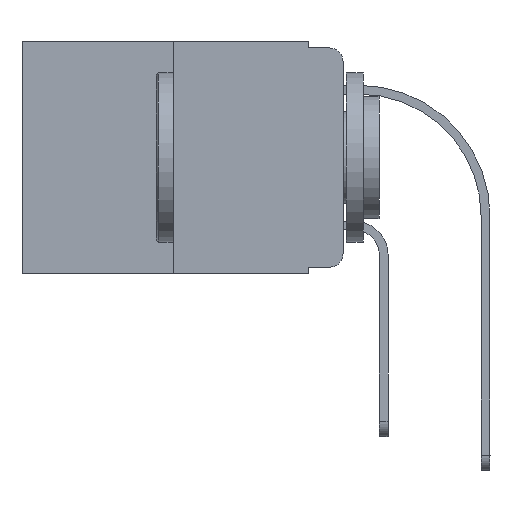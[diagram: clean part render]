
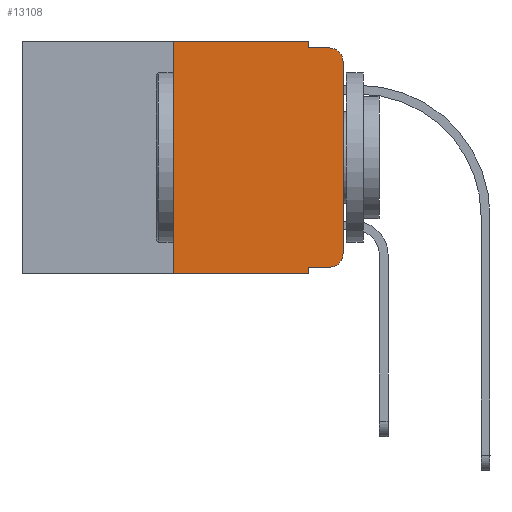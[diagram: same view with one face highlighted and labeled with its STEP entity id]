
A CAD part, left-side view. The second image highlights one B-rep face of the part: STEP entity #13108.
In plain terms, the highlighted planar face has unit normal (-1, 0, 0).
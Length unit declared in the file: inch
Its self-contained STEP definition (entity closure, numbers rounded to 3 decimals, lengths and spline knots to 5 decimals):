
#134 = DIRECTION ( 'NONE',  ( -1., 0., 0. ) ) ;
#656 = CARTESIAN_POINT ( 'NONE',  ( 0., 0., 0. ) ) ;
#934 = LINE ( 'NONE', #22986, #14768 ) ;
#983 = DIRECTION ( 'NONE',  ( 0., 0., -1. ) ) ;
#1268 = CARTESIAN_POINT ( 'NONE',  ( 0., 0.02, -0.01 ) ) ;
#1483 = VERTEX_POINT ( 'NONE', #3713 ) ;
#1506 = ORIENTED_EDGE ( 'NONE', *, *, #1952, .F. ) ;
#1589 = EDGE_CURVE ( 'NONE', #25586, #20872, #22453, .T. ) ;
#1952 = EDGE_CURVE ( 'NONE', #13489, #4452, #24661, .T. ) ;
#2121 = ORIENTED_EDGE ( 'NONE', *, *, #23318, .T. ) ;
#2332 = VERTEX_POINT ( 'NONE', #23731 ) ;
#2620 = DIRECTION ( 'NONE',  ( 0., -1., 0. ) ) ;
#2727 = DIRECTION ( 'NONE',  ( 0., -1., 0. ) ) ;
#2766 = CARTESIAN_POINT ( 'NONE',  ( 0., 0.051, -0.343 ) ) ;
#2879 = EDGE_CURVE ( 'NONE', #1483, #2332, #934, .T. ) ;
#3306 = ORIENTED_EDGE ( 'NONE', *, *, #19057, .F. ) ;
#3397 = VERTEX_POINT ( 'NONE', #7104 ) ;
#3544 = LINE ( 'NONE', #13345, #23094 ) ;
#3713 = CARTESIAN_POINT ( 'NONE',  ( 0., 0.051, -0.333 ) ) ;
#3762 = LINE ( 'NONE', #15770, #24955 ) ;
#3876 = FACE_OUTER_BOUND ( 'NONE', #21257, .T. ) ;
#3999 = CARTESIAN_POINT ( 'NONE',  ( 0., 0., -0.313 ) ) ;
#4319 = LINE ( 'NONE', #12385, #13441 ) ;
#4452 = VERTEX_POINT ( 'NONE', #1268 ) ;
#4532 = EDGE_CURVE ( 'NONE', #3397, #25586, #3762, .T. ) ;
#4614 = CARTESIAN_POINT ( 'NONE',  ( 0., 0.473, 0. ) ) ;
#6674 = CARTESIAN_POINT ( 'NONE',  ( 0., 0.25, 0. ) ) ;
#7056 = EDGE_CURVE ( 'NONE', #10008, #17159, #22970, .T. ) ;
#7104 = CARTESIAN_POINT ( 'NONE',  ( 0., 0.25, -0.343 ) ) ;
#7931 = CARTESIAN_POINT ( 'NONE',  ( 0., 0.02, -0.03 ) ) ;
#8430 = VERTEX_POINT ( 'NONE', #2766 ) ;
#8568 = DIRECTION ( 'NONE',  ( 0., 0., 1. ) ) ;
#9187 = EDGE_CURVE ( 'NONE', #20872, #13489, #4319, .T. ) ;
#9747 = ORIENTED_EDGE ( 'NONE', *, *, #4532, .F. ) ;
#10008 = VERTEX_POINT ( 'NONE', #3999 ) ;
#10447 = EDGE_CURVE ( 'NONE', #17159, #4452, #15920, .T. ) ;
#10716 = ORIENTED_EDGE ( 'NONE', *, *, #22805, .T. ) ;
#11942 = CARTESIAN_POINT ( 'NONE',  ( 0., 0.473, 0. ) ) ;
#12198 = DIRECTION ( 'NONE',  ( 1., 0., 0. ) ) ;
#12385 = CARTESIAN_POINT ( 'NONE',  ( 0., 0.051, 0. ) ) ;
#12400 = ORIENTED_EDGE ( 'NONE', *, *, #10447, .T. ) ;
#12424 = DIRECTION ( 'NONE',  ( 0., -1., 0. ) ) ;
#12690 = DIRECTION ( 'NONE',  ( 0., -1., 0. ) ) ;
#13108 = ADVANCED_FACE ( 'NONE', ( #3876 ), #20387, .F. ) ;
#13345 = CARTESIAN_POINT ( 'NONE',  ( 0., 0.051, 0. ) ) ;
#13441 = VECTOR ( 'NONE', #20444, 39.37008 ) ;
#13489 = VERTEX_POINT ( 'NONE', #18238 ) ;
#13525 = DIRECTION ( 'NONE',  ( -1., 0., 0. ) ) ;
#14381 = CARTESIAN_POINT ( 'NONE',  ( 0., 0.051, -0.01 ) ) ;
#14534 = VECTOR ( 'NONE', #2727, 39.37008 ) ;
#14768 = VECTOR ( 'NONE', #12424, 39.37008 ) ;
#15210 = CARTESIAN_POINT ( 'NONE',  ( 0., 0., -0.03 ) ) ;
#15311 = DIRECTION ( 'NONE',  ( 0., 0., -1. ) ) ;
#15389 = ORIENTED_EDGE ( 'NONE', *, *, #7056, .T. ) ;
#15740 = ORIENTED_EDGE ( 'NONE', *, *, #1589, .F. ) ;
#15770 = CARTESIAN_POINT ( 'NONE',  ( 0., 0.25, 0. ) ) ;
#15919 = CARTESIAN_POINT ( 'NONE',  ( 0., 0.051, 0. ) ) ;
#15920 = CIRCLE ( 'NONE', #16333, 0.02 ) ;
#16333 = AXIS2_PLACEMENT_3D ( 'NONE', #7931, #134, #20094 ) ;
#16717 = LINE ( 'NONE', #20815, #14534 ) ;
#17159 = VERTEX_POINT ( 'NONE', #15210 ) ;
#17491 = CIRCLE ( 'NONE', #20855, 0.02 ) ;
#18238 = CARTESIAN_POINT ( 'NONE',  ( 0., 0.051, -0.01 ) ) ;
#19057 = EDGE_CURVE ( 'NONE', #1483, #8430, #3544, .T. ) ;
#19744 = ORIENTED_EDGE ( 'NONE', *, *, #2879, .T. ) ;
#20094 = DIRECTION ( 'NONE',  ( 0., 0., -1. ) ) ;
#20387 = PLANE ( 'NONE',  #21940 ) ;
#20444 = DIRECTION ( 'NONE',  ( 0., 0., -1. ) ) ;
#20815 = CARTESIAN_POINT ( 'NONE',  ( 0., 0.473, -0.343 ) ) ;
#20855 = AXIS2_PLACEMENT_3D ( 'NONE', #23308, #13525, #983 ) ;
#20872 = VERTEX_POINT ( 'NONE', #15919 ) ;
#21091 = VECTOR ( 'NONE', #12690, 39.37008 ) ;
#21257 = EDGE_LOOP ( 'NONE', ( #15389, #12400, #1506, #25515, #15740, #9747, #10716, #3306, #19744, #2121 ) ) ;
#21940 = AXIS2_PLACEMENT_3D ( 'NONE', #11942, #12198, #22490 ) ;
#22453 = LINE ( 'NONE', #4614, #21091 ) ;
#22490 = DIRECTION ( 'NONE',  ( 0., 0., -1. ) ) ;
#22805 = EDGE_CURVE ( 'NONE', #3397, #8430, #16717, .T. ) ;
#22970 = LINE ( 'NONE', #656, #23488 ) ;
#22986 = CARTESIAN_POINT ( 'NONE',  ( 0., 0.051, -0.333 ) ) ;
#23094 = VECTOR ( 'NONE', #15311, 39.37008 ) ;
#23179 = VECTOR ( 'NONE', #2620, 39.37008 ) ;
#23308 = CARTESIAN_POINT ( 'NONE',  ( 0., 0.02, -0.313 ) ) ;
#23318 = EDGE_CURVE ( 'NONE', #2332, #10008, #17491, .T. ) ;
#23488 = VECTOR ( 'NONE', #8568, 39.37008 ) ;
#23731 = CARTESIAN_POINT ( 'NONE',  ( 0., 0.02, -0.333 ) ) ;
#23834 = DIRECTION ( 'NONE',  ( 0., 0., 1. ) ) ;
#24661 = LINE ( 'NONE', #14381, #23179 ) ;
#24955 = VECTOR ( 'NONE', #23834, 39.37008 ) ;
#25515 = ORIENTED_EDGE ( 'NONE', *, *, #9187, .F. ) ;
#25586 = VERTEX_POINT ( 'NONE', #6674 ) ;
